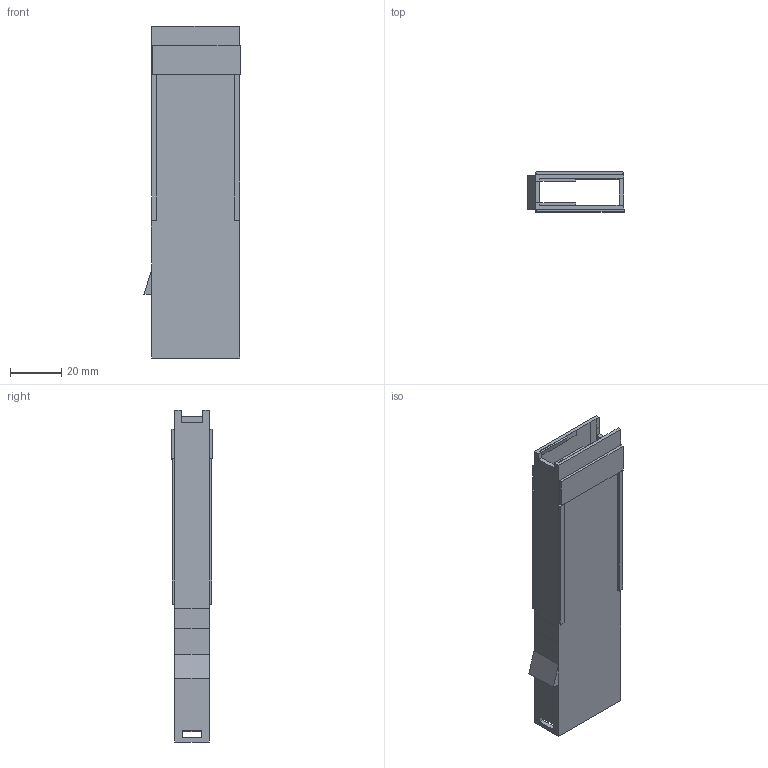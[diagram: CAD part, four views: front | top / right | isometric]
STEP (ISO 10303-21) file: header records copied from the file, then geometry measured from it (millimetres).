
FILE_DESCRIPTION(('FreeCAD Model'),'2;1');
FILE_NAME('magazine.step', '2015-07-10T13:24:53',('Author'),(''), 'Open CASCADE STEP processor 6.8','FreeCAD','Unknown');
FILE_SCHEMA(('AUTOMOTIVE_DESIGN_CC2 { 1 2 10303 214 -1 1 5 4 }'));
Length unit declared in the file: millimetre
Products named in the file (1): Pad013
Bounding box: 37.66 x 15.7 x 130 mm (x, y, z)
Volume: 19480.1 mm3; surface area: 24168 mm2
Topology: 1 solids, 1 shells, 108 faces, 296 edges, 188 vertices
Faces by surface type: plane 108
Entity records: 7066 total; most frequent: CARTESIAN_POINT 1316, DIRECTION 975, LINE 757, VECTOR 757, ORIENTED_EDGE 592, PCURVE 592, DEFINITIONAL_REPRESENTATION 592, EDGE_CURVE 296
